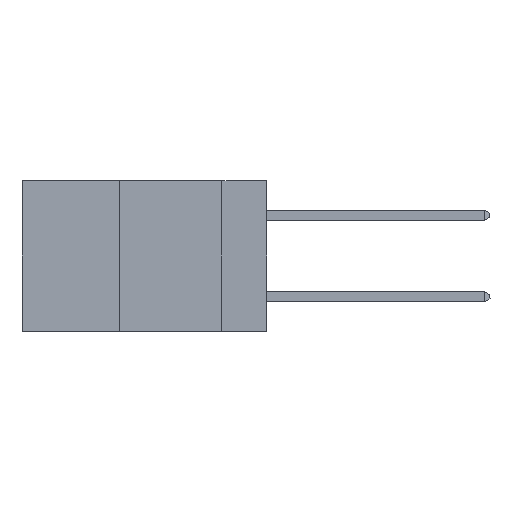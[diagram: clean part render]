
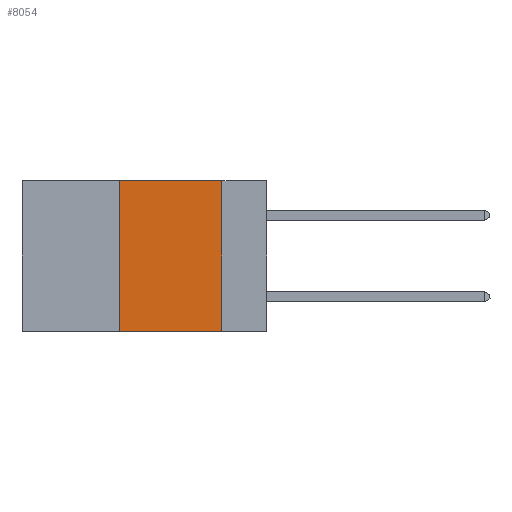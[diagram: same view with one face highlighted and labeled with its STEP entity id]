
A CAD part, left-side view. The second image highlights one B-rep face of the part: STEP entity #8054.
In plain terms, the highlighted planar face has unit normal (-1, 0, 0).
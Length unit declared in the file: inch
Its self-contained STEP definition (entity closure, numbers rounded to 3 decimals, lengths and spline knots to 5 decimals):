
#426 = DIRECTION ( 'NONE',  ( 0., 0., -1. ) ) ;
#715 = CARTESIAN_POINT ( 'NONE',  ( 0., 0.11, -0.37 ) ) ;
#1057 = EDGE_CURVE ( 'NONE', #1913, #4877, #14940, .T. ) ;
#1690 = EDGE_CURVE ( 'NONE', #4877, #3811, #3547, .T. ) ;
#1913 = VERTEX_POINT ( 'NONE', #14376 ) ;
#2170 = LINE ( 'NONE', #7920, #9557 ) ;
#3504 = ORIENTED_EDGE ( 'NONE', *, *, #16851, .F. ) ;
#3547 = LINE ( 'NONE', #11523, #8008 ) ;
#3566 = ORIENTED_EDGE ( 'NONE', *, *, #4415, .T. ) ;
#3811 = VERTEX_POINT ( 'NONE', #7795 ) ;
#4415 = EDGE_CURVE ( 'NONE', #1913, #17232, #2170, .T. ) ;
#4729 = CARTESIAN_POINT ( 'NONE',  ( 0., 0.36, 0. ) ) ;
#4877 = VERTEX_POINT ( 'NONE', #16608 ) ;
#6080 = EDGE_LOOP ( 'NONE', ( #3504, #8462, #12007, #3566 ) ) ;
#6786 = VECTOR ( 'NONE', #11803, 39.37008 ) ;
#6839 = DIRECTION ( 'NONE',  ( 0., 0., -1. ) ) ;
#7003 = DIRECTION ( 'NONE',  ( 1., 0., 0. ) ) ;
#7358 = DIRECTION ( 'NONE',  ( 0., -1., 0. ) ) ;
#7761 = VECTOR ( 'NONE', #6839, 39.37008 ) ;
#7795 = CARTESIAN_POINT ( 'NONE',  ( 0., 0.11, 0. ) ) ;
#7920 = CARTESIAN_POINT ( 'NONE',  ( 0., 0.6, -0.37 ) ) ;
#8008 = VECTOR ( 'NONE', #7358, 39.37008 ) ;
#8054 = ADVANCED_FACE ( 'NONE', ( #17400 ), #11110, .F. ) ;
#8462 = ORIENTED_EDGE ( 'NONE', *, *, #1690, .F. ) ;
#9202 = LINE ( 'NONE', #13514, #7761 ) ;
#9557 = VECTOR ( 'NONE', #17283, 39.37008 ) ;
#11110 = PLANE ( 'NONE',  #16988 ) ;
#11523 = CARTESIAN_POINT ( 'NONE',  ( 0., 0.6, 0. ) ) ;
#11803 = DIRECTION ( 'NONE',  ( 0., 0., 1. ) ) ;
#12007 = ORIENTED_EDGE ( 'NONE', *, *, #1057, .F. ) ;
#13514 = CARTESIAN_POINT ( 'NONE',  ( 0., 0.11, 0. ) ) ;
#13681 = CARTESIAN_POINT ( 'NONE',  ( 0., 0.6, 0. ) ) ;
#14376 = CARTESIAN_POINT ( 'NONE',  ( 0., 0.36, -0.37 ) ) ;
#14940 = LINE ( 'NONE', #4729, #6786 ) ;
#16608 = CARTESIAN_POINT ( 'NONE',  ( 0., 0.36, 0. ) ) ;
#16851 = EDGE_CURVE ( 'NONE', #3811, #17232, #9202, .T. ) ;
#16988 = AXIS2_PLACEMENT_3D ( 'NONE', #13681, #7003, #426 ) ;
#17232 = VERTEX_POINT ( 'NONE', #715 ) ;
#17283 = DIRECTION ( 'NONE',  ( 0., -1., 0. ) ) ;
#17400 = FACE_OUTER_BOUND ( 'NONE', #6080, .T. ) ;
